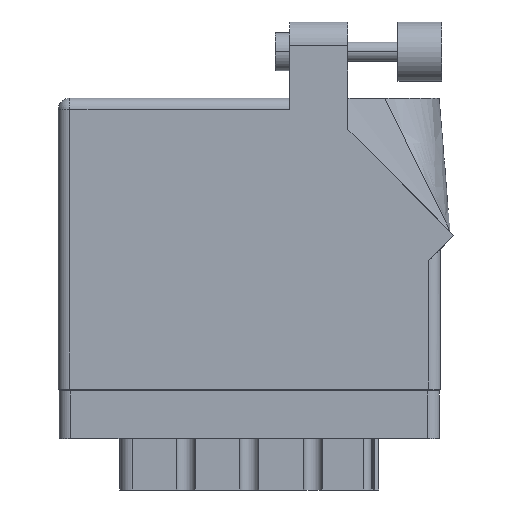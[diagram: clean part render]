
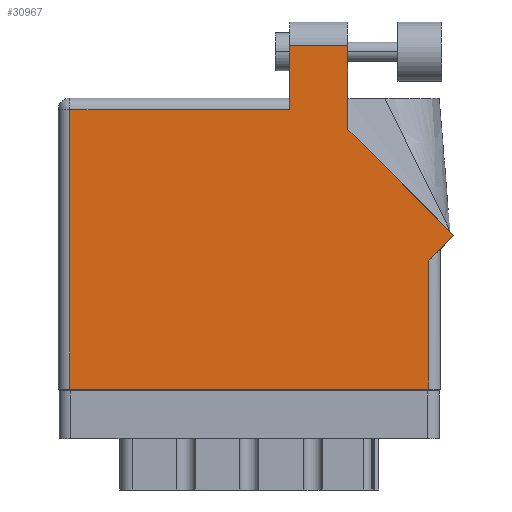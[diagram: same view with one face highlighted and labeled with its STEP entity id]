
A CAD part, front view. The second image highlights one B-rep face of the part: STEP entity #30967.
In plain terms, the highlighted face is planar.
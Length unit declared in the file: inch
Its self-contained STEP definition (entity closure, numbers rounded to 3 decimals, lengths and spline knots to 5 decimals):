
#49 = EDGE_CURVE ( 'NONE', #26886, #22034, #30231, .T. ) ;
#211 = CARTESIAN_POINT ( 'NONE',  ( 1.524, 1.36442, 0. ) ) ;
#474 = VECTOR ( 'NONE', #35573, 39.37008 ) ;
#554 = CARTESIAN_POINT ( 'NONE',  ( 1.948, 0., 0. ) ) ;
#1291 = CARTESIAN_POINT ( 'NONE',  ( 0.062, 0., 0. ) ) ;
#1355 = VECTOR ( 'NONE', #31777, 39.37008 ) ;
#2062 = LINE ( 'NONE', #10792, #21034 ) ;
#2445 = VERTEX_POINT ( 'NONE', #1291 ) ;
#2857 = DIRECTION ( 'NONE',  ( 0., 1., 0. ) ) ;
#3264 = CARTESIAN_POINT ( 'NONE',  ( 0., 0., 0. ) ) ;
#3295 = VECTOR ( 'NONE', #26323, 39.37008 ) ;
#3782 = VECTOR ( 'NONE', #35377, 39.37008 ) ;
#3810 = LINE ( 'NONE', #4323, #10591 ) ;
#3885 = VECTOR ( 'NONE', #22071, 39.37008 ) ;
#4323 = CARTESIAN_POINT ( 'NONE',  ( 1.948, 0.737, 0. ) ) ;
#4606 = VERTEX_POINT ( 'NONE', #554 ) ;
#4825 = EDGE_CURVE ( 'NONE', #4606, #33292, #3810, .T. ) ;
#5610 = CARTESIAN_POINT ( 'NONE',  ( 1.948, 0.675, 0. ) ) ;
#5793 = VERTEX_POINT ( 'NONE', #26066 ) ;
#6058 = FACE_OUTER_BOUND ( 'NONE', #28382, .T. ) ;
#6914 = CARTESIAN_POINT ( 'NONE',  ( 0.062, 0., 0. ) ) ;
#8198 = VERTEX_POINT ( 'NONE', #30474 ) ;
#8584 = LINE ( 'NONE', #20128, #1355 ) ;
#9193 = CARTESIAN_POINT ( 'NONE',  ( 2.01, 0.737, 0. ) ) ;
#10412 = ORIENTED_EDGE ( 'NONE', *, *, #4825, .T. ) ;
#10591 = VECTOR ( 'NONE', #24627, 39.37008 ) ;
#10792 = CARTESIAN_POINT ( 'NONE',  ( 1.217, 1.805, 0. ) ) ;
#11747 = DIRECTION ( 'NONE',  ( 0.707, 0.707, 0. ) ) ;
#13385 = CARTESIAN_POINT ( 'NONE',  ( 1.217, 1.53, 0. ) ) ;
#13495 = ORIENTED_EDGE ( 'NONE', *, *, #34977, .T. ) ;
#14316 = LINE ( 'NONE', #13385, #3885 ) ;
#15507 = EDGE_CURVE ( 'NONE', #22034, #8198, #2062, .T. ) ;
#16392 = DIRECTION ( 'NONE',  ( -1., 0., 0. ) ) ;
#19785 = VERTEX_POINT ( 'NONE', #25870 ) ;
#19977 = LINE ( 'NONE', #3264, #3295 ) ;
#20128 = CARTESIAN_POINT ( 'NONE',  ( 2.08071, 0.80771, 0. ) ) ;
#20138 = CARTESIAN_POINT ( 'NONE',  ( 1.524, 1.36442, 0. ) ) ;
#21034 = VECTOR ( 'NONE', #34309, 39.37008 ) ;
#21164 = ORIENTED_EDGE ( 'NONE', *, *, #36722, .T. ) ;
#21713 = VECTOR ( 'NONE', #2857, 39.37008 ) ;
#22034 = VERTEX_POINT ( 'NONE', #31530 ) ;
#22042 = ORIENTED_EDGE ( 'NONE', *, *, #34444, .T. ) ;
#22071 = DIRECTION ( 'NONE',  ( 0., -1., 0. ) ) ;
#24048 = VERTEX_POINT ( 'NONE', #28130 ) ;
#24331 = EDGE_CURVE ( 'NONE', #33292, #5793, #37226, .T. ) ;
#24571 = AXIS2_PLACEMENT_3D ( 'NONE', #28077, #33592, #16392 ) ;
#24627 = DIRECTION ( 'NONE',  ( 0., 1., 0. ) ) ;
#24750 = ORIENTED_EDGE ( 'NONE', *, *, #15507, .T. ) ;
#25870 = CARTESIAN_POINT ( 'NONE',  ( 0.062, 1.468, 0. ) ) ;
#26066 = CARTESIAN_POINT ( 'NONE',  ( 2.08071, 0.80771, 0. ) ) ;
#26323 = DIRECTION ( 'NONE',  ( 1., 0., 0. ) ) ;
#26847 = EDGE_CURVE ( 'NONE', #19785, #2445, #28009, .T. ) ;
#26886 = VERTEX_POINT ( 'NONE', #211 ) ;
#27209 = EDGE_CURVE ( 'NONE', #5793, #26886, #8584, .T. ) ;
#28009 = LINE ( 'NONE', #6914, #474 ) ;
#28072 = ORIENTED_EDGE ( 'NONE', *, *, #27209, .T. ) ;
#28077 = CARTESIAN_POINT ( 'NONE',  ( 0., 1.53, 0. ) ) ;
#28130 = CARTESIAN_POINT ( 'NONE',  ( 1.217, 1.468, 0. ) ) ;
#28382 = EDGE_LOOP ( 'NONE', ( #36790, #24750, #21164, #22042, #33722, #13495, #10412, #35899, #28072 ) ) ;
#30231 = LINE ( 'NONE', #20138, #21713 ) ;
#30474 = CARTESIAN_POINT ( 'NONE',  ( 1.217, 1.805, 0. ) ) ;
#30688 = PLANE ( 'NONE',  #24571 ) ;
#30967 = ADVANCED_FACE ( 'NONE', ( #6058 ), #30688, .F. ) ;
#31530 = CARTESIAN_POINT ( 'NONE',  ( 1.524, 1.805, 0. ) ) ;
#31777 = DIRECTION ( 'NONE',  ( -0.707, 0.707, 0. ) ) ;
#32606 = CARTESIAN_POINT ( 'NONE',  ( 0., 1.468, 0. ) ) ;
#33292 = VERTEX_POINT ( 'NONE', #5610 ) ;
#33592 = DIRECTION ( 'NONE',  ( 0., 0., -1. ) ) ;
#33722 = ORIENTED_EDGE ( 'NONE', *, *, #26847, .T. ) ;
#33952 = LINE ( 'NONE', #32606, #3782 ) ;
#34309 = DIRECTION ( 'NONE',  ( -1., 0., 0. ) ) ;
#34444 = EDGE_CURVE ( 'NONE', #24048, #19785, #33952, .T. ) ;
#34977 = EDGE_CURVE ( 'NONE', #2445, #4606, #19977, .T. ) ;
#35377 = DIRECTION ( 'NONE',  ( -1., 0., 0. ) ) ;
#35385 = VECTOR ( 'NONE', #11747, 39.37008 ) ;
#35573 = DIRECTION ( 'NONE',  ( 0., -1., 0. ) ) ;
#35899 = ORIENTED_EDGE ( 'NONE', *, *, #24331, .T. ) ;
#36722 = EDGE_CURVE ( 'NONE', #8198, #24048, #14316, .T. ) ;
#36790 = ORIENTED_EDGE ( 'NONE', *, *, #49, .T. ) ;
#37226 = LINE ( 'NONE', #9193, #35385 ) ;
